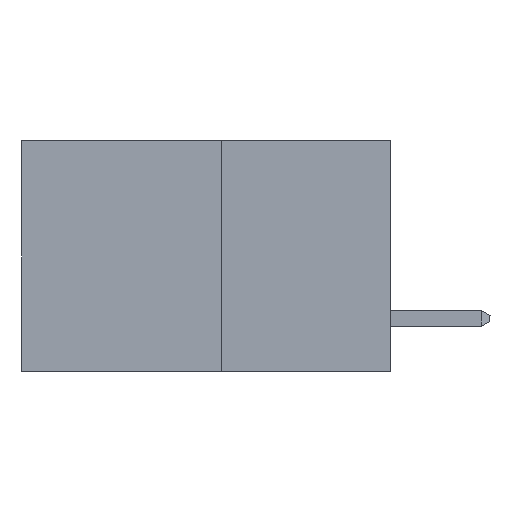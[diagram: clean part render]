
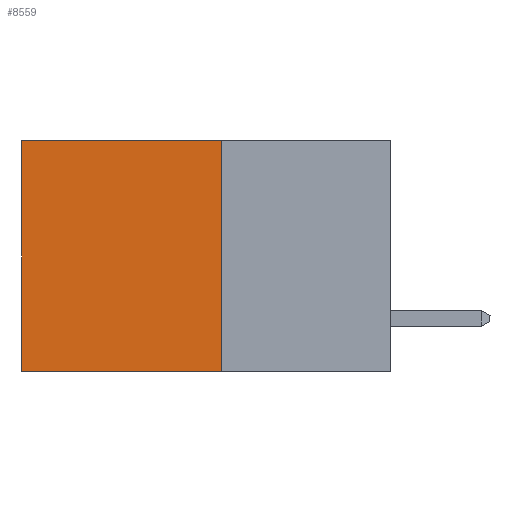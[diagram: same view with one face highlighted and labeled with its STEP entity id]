
A CAD part, left-side view. The second image highlights one B-rep face of the part: STEP entity #8559.
In plain terms, the highlighted planar face has unit normal (-1, 0, 0).
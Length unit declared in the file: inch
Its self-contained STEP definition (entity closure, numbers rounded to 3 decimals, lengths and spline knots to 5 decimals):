
#655 = VERTEX_POINT ( 'NONE', #32375 ) ;
#3906 = VERTEX_POINT ( 'NONE', #19981 ) ;
#4064 = EDGE_LOOP ( 'NONE', ( #6571, #31630, #23287, #14073 ) ) ;
#5163 = CARTESIAN_POINT ( 'NONE',  ( 0.277, 0.27, -0.37 ) ) ;
#6571 = ORIENTED_EDGE ( 'NONE', *, *, #18377, .T. ) ;
#8559 = ADVANCED_FACE ( 'NONE', ( #19484 ), #9750, .F. ) ;
#9750 = PLANE ( 'NONE',  #11717 ) ;
#10518 = LINE ( 'NONE', #31129, #24574 ) ;
#10816 = VERTEX_POINT ( 'NONE', #13580 ) ;
#11009 = DIRECTION ( 'NONE',  ( 0., 1., 0. ) ) ;
#11300 = VECTOR ( 'NONE', #11009, 39.37008 ) ;
#11717 = AXIS2_PLACEMENT_3D ( 'NONE', #33674, #11992, #14688 ) ;
#11992 = DIRECTION ( 'NONE',  ( 1., 0., 0. ) ) ;
#13531 = EDGE_CURVE ( 'NONE', #20218, #655, #30534, .T. ) ;
#13580 = CARTESIAN_POINT ( 'NONE',  ( 0.277, 0.59, 0. ) ) ;
#14073 = ORIENTED_EDGE ( 'NONE', *, *, #19184, .T. ) ;
#14688 = DIRECTION ( 'NONE',  ( 0., 0., -1. ) ) ;
#16231 = CARTESIAN_POINT ( 'NONE',  ( 0.277, 0.27, 0. ) ) ;
#17663 = CARTESIAN_POINT ( 'NONE',  ( 0.277, 0.27, 0. ) ) ;
#17882 = DIRECTION ( 'NONE',  ( 0., 0., -1. ) ) ;
#18347 = LINE ( 'NONE', #16231, #11300 ) ;
#18377 = EDGE_CURVE ( 'NONE', #10816, #3906, #10518, .T. ) ;
#18925 = VECTOR ( 'NONE', #22987, 39.37008 ) ;
#19184 = EDGE_CURVE ( 'NONE', #20218, #10816, #18347, .T. ) ;
#19484 = FACE_OUTER_BOUND ( 'NONE', #4064, .T. ) ;
#19981 = CARTESIAN_POINT ( 'NONE',  ( 0.277, 0.59, -0.37 ) ) ;
#20218 = VERTEX_POINT ( 'NONE', #17663 ) ;
#22987 = DIRECTION ( 'NONE',  ( 0., 0., -1. ) ) ;
#23057 = CARTESIAN_POINT ( 'NONE',  ( 0.277, 0.27, -0.37 ) ) ;
#23287 = ORIENTED_EDGE ( 'NONE', *, *, #13531, .F. ) ;
#24022 = EDGE_CURVE ( 'NONE', #655, #3906, #34336, .T. ) ;
#24574 = VECTOR ( 'NONE', #17882, 39.37008 ) ;
#27217 = VECTOR ( 'NONE', #29072, 39.37008 ) ;
#29072 = DIRECTION ( 'NONE',  ( 0., 1., 0. ) ) ;
#30534 = LINE ( 'NONE', #23057, #18925 ) ;
#31129 = CARTESIAN_POINT ( 'NONE',  ( 0.277, 0.59, -0.37 ) ) ;
#31630 = ORIENTED_EDGE ( 'NONE', *, *, #24022, .F. ) ;
#32375 = CARTESIAN_POINT ( 'NONE',  ( 0.277, 0.27, -0.37 ) ) ;
#33674 = CARTESIAN_POINT ( 'NONE',  ( 0.277, 0.27, -0.37 ) ) ;
#34336 = LINE ( 'NONE', #5163, #27217 ) ;
